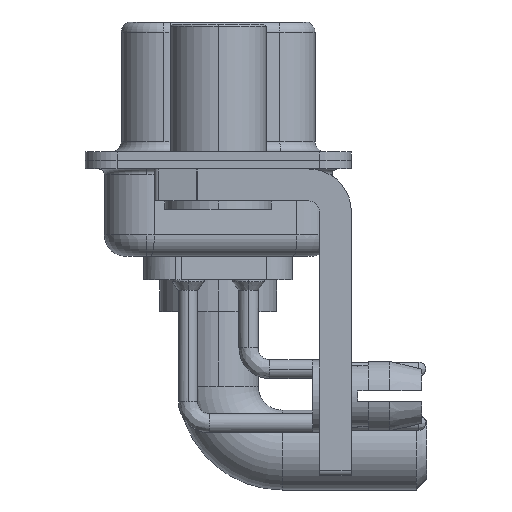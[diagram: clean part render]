
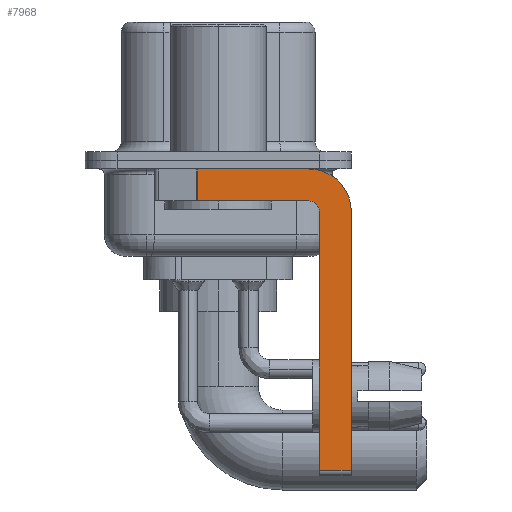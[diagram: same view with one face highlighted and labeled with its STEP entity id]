
A CAD part, left-side view. The second image highlights one B-rep face of the part: STEP entity #7968.
In plain terms, the highlighted planar face has unit normal (-1, 0, 0).
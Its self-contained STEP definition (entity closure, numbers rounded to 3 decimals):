
#106 = FACE_OUTER_BOUND ( 'NONE', #12273, .T. ) ;
#362 = CARTESIAN_POINT ( 'NONE',  ( -2.9, -4.25, -0.4 ) ) ;
#1582 = DIRECTION ( 'NONE',  ( 0., -1., 0. ) ) ;
#2296 = LINE ( 'NONE', #6364, #7616 ) ;
#3226 = VECTOR ( 'NONE', #3863, 1000. ) ;
#3741 = AXIS2_PLACEMENT_3D ( 'NONE', #5707, #7794, #9364 ) ;
#3863 = DIRECTION ( 'NONE',  ( 0., 0., -1. ) ) ;
#4115 = VERTEX_POINT ( 'NONE', #13476 ) ;
#4346 = CARTESIAN_POINT ( 'NONE',  ( -2.9, 0.978, -1.9 ) ) ;
#5283 = ORIENTED_EDGE ( 'NONE', *, *, #6056, .T. ) ;
#5516 = DIRECTION ( 'NONE',  ( 0., -1., 0. ) ) ;
#5707 = CARTESIAN_POINT ( 'NONE',  ( -2.9, -4.25, -2.4 ) ) ;
#6056 = EDGE_CURVE ( 'NONE', #12774, #20314, #16767, .T. ) ;
#6364 = CARTESIAN_POINT ( 'NONE',  ( -2.9, -4.75, -14.8 ) ) ;
#6461 = DIRECTION ( 'NONE',  ( 0., 1., 0. ) ) ;
#6816 = DIRECTION ( 'NONE',  ( 0., 0., -1. ) ) ;
#7616 = VECTOR ( 'NONE', #16568, 1000. ) ;
#7794 = DIRECTION ( 'NONE',  ( 1., 0., 0. ) ) ;
#7847 = CARTESIAN_POINT ( 'NONE',  ( -2.9, -4.25, -2.4 ) ) ;
#7968 = ADVANCED_FACE ( 'NONE', ( #106 ), #11644, .F. ) ;
#8930 = LINE ( 'NONE', #14838, #22677 ) ;
#9364 = DIRECTION ( 'NONE',  ( 0., 0., -1. ) ) ;
#10841 = ORIENTED_EDGE ( 'NONE', *, *, #12278, .F. ) ;
#11257 = CARTESIAN_POINT ( 'NONE',  ( -2.9, -6.25, -14.55 ) ) ;
#11349 = CARTESIAN_POINT ( 'NONE',  ( -2.9, 0.978, -1.9 ) ) ;
#11402 = VECTOR ( 'NONE', #1582, 1000. ) ;
#11644 = PLANE ( 'NONE',  #13076 ) ;
#11959 = CARTESIAN_POINT ( 'NONE',  ( -2.9, -6.25, -2.4 ) ) ;
#12273 = EDGE_LOOP ( 'NONE', ( #17736, #5283, #12646, #20009, #10841, #14698, #15135, #14564 ) ) ;
#12278 = EDGE_CURVE ( 'NONE', #4115, #23760, #2296, .T. ) ;
#12646 = ORIENTED_EDGE ( 'NONE', *, *, #14360, .F. ) ;
#12774 = VERTEX_POINT ( 'NONE', #18226 ) ;
#13076 = AXIS2_PLACEMENT_3D ( 'NONE', #7847, #13494, #14008 ) ;
#13476 = CARTESIAN_POINT ( 'NONE',  ( -2.9, -4.75, -14.55 ) ) ;
#13494 = DIRECTION ( 'NONE',  ( 1., 0., 0. ) ) ;
#14008 = DIRECTION ( 'NONE',  ( 0., 0., -1. ) ) ;
#14297 = VECTOR ( 'NONE', #6816, 1000. ) ;
#14360 = EDGE_CURVE ( 'NONE', #16148, #20314, #8930, .T. ) ;
#14442 = EDGE_CURVE ( 'NONE', #12774, #21736, #23327, .T. ) ;
#14564 = ORIENTED_EDGE ( 'NONE', *, *, #22478, .F. ) ;
#14698 = ORIENTED_EDGE ( 'NONE', *, *, #22860, .T. ) ;
#14838 = CARTESIAN_POINT ( 'NONE',  ( -2.9, -4.25, -1.9 ) ) ;
#15056 = EDGE_CURVE ( 'NONE', #23760, #16148, #24797, .T. ) ;
#15106 = CARTESIAN_POINT ( 'NONE',  ( -2.9, 3., -0.4 ) ) ;
#15135 = ORIENTED_EDGE ( 'NONE', *, *, #19334, .F. ) ;
#16148 = VERTEX_POINT ( 'NONE', #20685 ) ;
#16200 = CARTESIAN_POINT ( 'NONE',  ( -2.9, -4.25, -2.4 ) ) ;
#16462 = AXIS2_PLACEMENT_3D ( 'NONE', #16200, #24291, #18525 ) ;
#16568 = DIRECTION ( 'NONE',  ( 0., 0., 1. ) ) ;
#16599 = VERTEX_POINT ( 'NONE', #22872 ) ;
#16767 = LINE ( 'NONE', #11349, #14297 ) ;
#17425 = LINE ( 'NONE', #21085, #25851 ) ;
#17736 = ORIENTED_EDGE ( 'NONE', *, *, #14442, .F. ) ;
#18226 = CARTESIAN_POINT ( 'NONE',  ( -2.9, 0.978, -0.4 ) ) ;
#18327 = VERTEX_POINT ( 'NONE', #11257 ) ;
#18525 = DIRECTION ( 'NONE',  ( 0., 0., 1. ) ) ;
#19334 = EDGE_CURVE ( 'NONE', #16599, #18327, #21659, .T. ) ;
#20009 = ORIENTED_EDGE ( 'NONE', *, *, #15056, .F. ) ;
#20314 = VERTEX_POINT ( 'NONE', #4346 ) ;
#20685 = CARTESIAN_POINT ( 'NONE',  ( -2.9, -4.25, -1.9 ) ) ;
#20861 = CIRCLE ( 'NONE', #3741, 2. ) ;
#21085 = CARTESIAN_POINT ( 'NONE',  ( -2.9, -4.25, -14.55 ) ) ;
#21659 = LINE ( 'NONE', #11959, #3226 ) ;
#21736 = VERTEX_POINT ( 'NONE', #362 ) ;
#22478 = EDGE_CURVE ( 'NONE', #21736, #16599, #20861, .T. ) ;
#22677 = VECTOR ( 'NONE', #6461, 1000. ) ;
#22696 = CARTESIAN_POINT ( 'NONE',  ( -2.9, -4.75, -2.4 ) ) ;
#22860 = EDGE_CURVE ( 'NONE', #4115, #18327, #17425, .T. ) ;
#22872 = CARTESIAN_POINT ( 'NONE',  ( -2.9, -6.25, -2.4 ) ) ;
#23327 = LINE ( 'NONE', #15106, #11402 ) ;
#23760 = VERTEX_POINT ( 'NONE', #22696 ) ;
#24291 = DIRECTION ( 'NONE',  ( -1., 0., 0. ) ) ;
#24797 = CIRCLE ( 'NONE', #16462, 0.5 ) ;
#25851 = VECTOR ( 'NONE', #5516, 1000. ) ;
